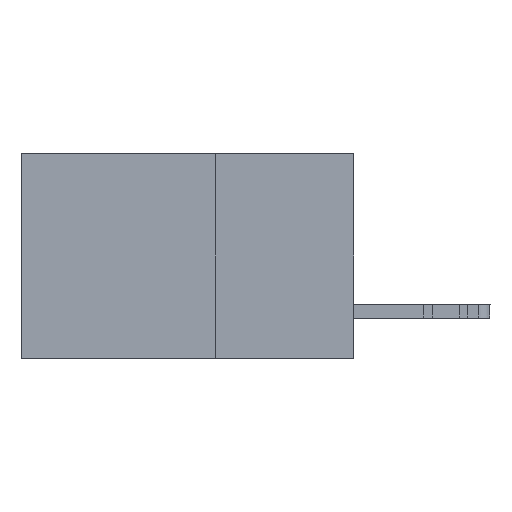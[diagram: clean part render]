
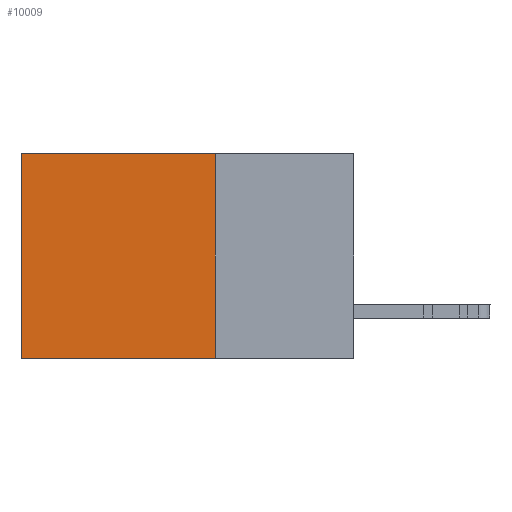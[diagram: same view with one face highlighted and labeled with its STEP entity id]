
A CAD part, left-side view. The second image highlights one B-rep face of the part: STEP entity #10009.
In plain terms, the highlighted planar face has unit normal (-1, 0, 0).
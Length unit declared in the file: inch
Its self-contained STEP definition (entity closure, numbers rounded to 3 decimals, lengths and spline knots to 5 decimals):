
#542 = VERTEX_POINT ( 'NONE', #22705 ) ;
#2113 = CARTESIAN_POINT ( 'NONE',  ( 0.2875, 0.25, 0. ) ) ;
#2271 = LINE ( 'NONE', #16582, #24279 ) ;
#4795 = ORIENTED_EDGE ( 'NONE', *, *, #13904, .T. ) ;
#6045 = CARTESIAN_POINT ( 'NONE',  ( 0.2875, 0.25, 0. ) ) ;
#10009 = ADVANCED_FACE ( 'NONE', ( #37522 ), #26734, .F. ) ;
#11743 = CARTESIAN_POINT ( 'NONE',  ( 0.2875, 0.25, -0.37 ) ) ;
#11783 = LINE ( 'NONE', #33343, #39863 ) ;
#13243 = LINE ( 'NONE', #45388, #21206 ) ;
#13904 = EDGE_CURVE ( 'NONE', #542, #40617, #13243, .T. ) ;
#16582 = CARTESIAN_POINT ( 'NONE',  ( 0.2875, 0.25, -0.37 ) ) ;
#19237 = VERTEX_POINT ( 'NONE', #11743 ) ;
#19702 = DIRECTION ( 'NONE',  ( 0., 0., -1. ) ) ;
#20009 = DIRECTION ( 'NONE',  ( 0., 0., -1. ) ) ;
#21206 = VECTOR ( 'NONE', #30835, 39.37008 ) ;
#22705 = CARTESIAN_POINT ( 'NONE',  ( 0.2875, 0.6, 0. ) ) ;
#23286 = LINE ( 'NONE', #37834, #38383 ) ;
#24133 = EDGE_CURVE ( 'NONE', #40820, #19237, #23286, .T. ) ;
#24279 = VECTOR ( 'NONE', #30889, 39.37008 ) ;
#25423 = EDGE_CURVE ( 'NONE', #40820, #542, #11783, .T. ) ;
#25998 = ORIENTED_EDGE ( 'NONE', *, *, #27785, .F. ) ;
#26734 = PLANE ( 'NONE',  #44152 ) ;
#27785 = EDGE_CURVE ( 'NONE', #19237, #40617, #2271, .T. ) ;
#30835 = DIRECTION ( 'NONE',  ( 0., 0., -1. ) ) ;
#30889 = DIRECTION ( 'NONE',  ( 0., 1., 0. ) ) ;
#31211 = ORIENTED_EDGE ( 'NONE', *, *, #24133, .F. ) ;
#33343 = CARTESIAN_POINT ( 'NONE',  ( 0.2875, 0.25, 0. ) ) ;
#34710 = DIRECTION ( 'NONE',  ( 1., 0., 0. ) ) ;
#37100 = DIRECTION ( 'NONE',  ( 0., 1., 0. ) ) ;
#37522 = FACE_OUTER_BOUND ( 'NONE', #39812, .T. ) ;
#37834 = CARTESIAN_POINT ( 'NONE',  ( 0.2875, 0.25, 0. ) ) ;
#38383 = VECTOR ( 'NONE', #20009, 39.37008 ) ;
#39812 = EDGE_LOOP ( 'NONE', ( #4795, #25998, #31211, #40367 ) ) ;
#39863 = VECTOR ( 'NONE', #37100, 39.37008 ) ;
#40367 = ORIENTED_EDGE ( 'NONE', *, *, #25423, .T. ) ;
#40617 = VERTEX_POINT ( 'NONE', #42469 ) ;
#40820 = VERTEX_POINT ( 'NONE', #6045 ) ;
#42469 = CARTESIAN_POINT ( 'NONE',  ( 0.2875, 0.6, -0.37 ) ) ;
#44152 = AXIS2_PLACEMENT_3D ( 'NONE', #2113, #34710, #19702 ) ;
#45388 = CARTESIAN_POINT ( 'NONE',  ( 0.2875, 0.6, 0. ) ) ;
